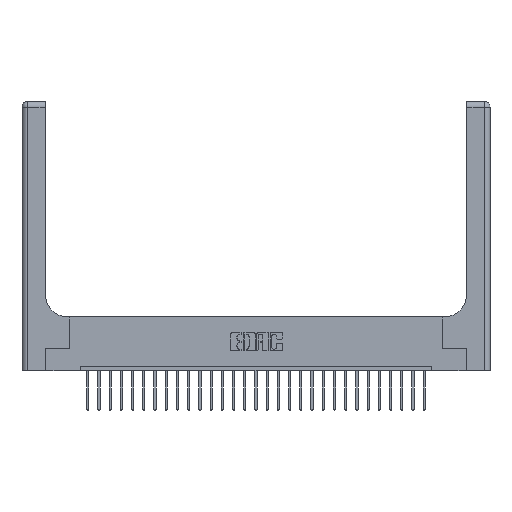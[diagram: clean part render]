
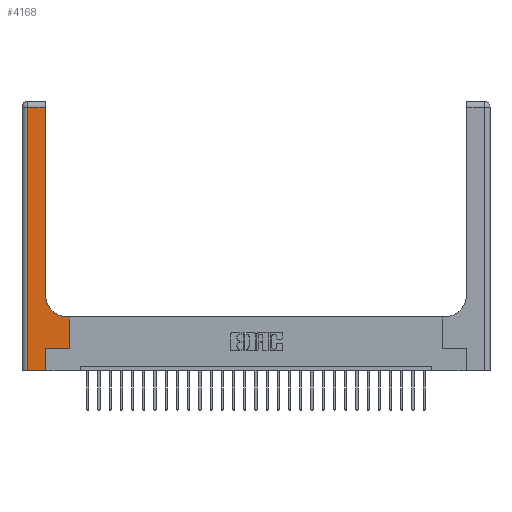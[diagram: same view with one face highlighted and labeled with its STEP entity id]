
A CAD part, top view. The second image highlights one B-rep face of the part: STEP entity #4168.
In plain terms, the highlighted planar face has unit normal (0, 0, 1).
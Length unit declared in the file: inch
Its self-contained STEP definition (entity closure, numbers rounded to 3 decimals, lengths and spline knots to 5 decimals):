
#510 = CARTESIAN_POINT ( 'NONE',  ( 0.26, 0.85, 0.37 ) ) ;
#938 = VERTEX_POINT ( 'NONE', #22805 ) ;
#1607 = LINE ( 'NONE', #25486, #23096 ) ;
#1623 = VECTOR ( 'NONE', #7981, 39.37008 ) ;
#1675 = DIRECTION ( 'NONE',  ( 0., 1., 0. ) ) ;
#1730 = CARTESIAN_POINT ( 'NONE',  ( 0., 0., 0.37 ) ) ;
#1995 = VERTEX_POINT ( 'NONE', #13888 ) ;
#2471 = DIRECTION ( 'NONE',  ( 0., 0., -1. ) ) ;
#3224 = VERTEX_POINT ( 'NONE', #7228 ) ;
#3388 = VERTEX_POINT ( 'NONE', #16816 ) ;
#3666 = CARTESIAN_POINT ( 'NONE',  ( 0.528, 0.25, 0.37 ) ) ;
#3952 = VERTEX_POINT ( 'NONE', #13189 ) ;
#4013 = CARTESIAN_POINT ( 'NONE',  ( 0.26, 0.6, 0.37 ) ) ;
#4091 = CARTESIAN_POINT ( 'NONE',  ( 0.26, 3., 0.37 ) ) ;
#4106 = EDGE_CURVE ( 'NONE', #938, #3388, #9564, .T. ) ;
#4168 = ADVANCED_FACE ( 'NONE', ( #8212 ), #18738, .F. ) ;
#5212 = DIRECTION ( 'NONE',  ( 1., 0., 0. ) ) ;
#5298 = EDGE_CURVE ( 'NONE', #1995, #7631, #5673, .T. ) ;
#5673 = LINE ( 'NONE', #19688, #8326 ) ;
#5877 = LINE ( 'NONE', #4013, #9491 ) ;
#6114 = VECTOR ( 'NONE', #1675, 39.37008 ) ;
#6427 = VERTEX_POINT ( 'NONE', #13700 ) ;
#6480 = EDGE_CURVE ( 'NONE', #9875, #25580, #8840, .T. ) ;
#7228 = CARTESIAN_POINT ( 'NONE',  ( 0.528, 0.25, 0.37 ) ) ;
#7511 = EDGE_CURVE ( 'NONE', #7631, #3952, #24387, .T. ) ;
#7631 = VERTEX_POINT ( 'NONE', #9044 ) ;
#7810 = DIRECTION ( 'NONE',  ( 0., 1., 0. ) ) ;
#7981 = DIRECTION ( 'NONE',  ( 0., -1., 0. ) ) ;
#8212 = FACE_OUTER_BOUND ( 'NONE', #10361, .T. ) ;
#8326 = VECTOR ( 'NONE', #15957, 39.37008 ) ;
#8474 = CARTESIAN_POINT ( 'NONE',  ( 0., 3., 0.37 ) ) ;
#8840 = CIRCLE ( 'NONE', #23749, 0.25 ) ;
#9044 = CARTESIAN_POINT ( 'NONE',  ( 0.06, 2.94, 0.37 ) ) ;
#9255 = EDGE_CURVE ( 'NONE', #25580, #1995, #10365, .T. ) ;
#9358 = VECTOR ( 'NONE', #22104, 39.37008 ) ;
#9491 = VECTOR ( 'NONE', #16160, 39.37008 ) ;
#9564 = LINE ( 'NONE', #26076, #21756 ) ;
#9875 = VERTEX_POINT ( 'NONE', #20998 ) ;
#10361 = EDGE_LOOP ( 'NONE', ( #24548, #23076, #20923, #11060, #18143, #10682, #15654, #11019, #11666 ) ) ;
#10365 = LINE ( 'NONE', #4091, #9358 ) ;
#10682 = ORIENTED_EDGE ( 'NONE', *, *, #14332, .T. ) ;
#11019 = ORIENTED_EDGE ( 'NONE', *, *, #20191, .T. ) ;
#11060 = ORIENTED_EDGE ( 'NONE', *, *, #25303, .T. ) ;
#11666 = ORIENTED_EDGE ( 'NONE', *, *, #6480, .T. ) ;
#11710 = DIRECTION ( 'NONE',  ( 1., 0., 0. ) ) ;
#11883 = DIRECTION ( 'NONE',  ( 1., 0., 0. ) ) ;
#11970 = CARTESIAN_POINT ( 'NONE',  ( 0.51, 0.85, 0.37 ) ) ;
#13189 = CARTESIAN_POINT ( 'NONE',  ( 0.06, 0., 0.37 ) ) ;
#13700 = CARTESIAN_POINT ( 'NONE',  ( 0.528, 0.6, 0.37 ) ) ;
#13888 = CARTESIAN_POINT ( 'NONE',  ( 0.26, 2.94, 0.37 ) ) ;
#14332 = EDGE_CURVE ( 'NONE', #3388, #3224, #1607, .T. ) ;
#15654 = ORIENTED_EDGE ( 'NONE', *, *, #20967, .T. ) ;
#15957 = DIRECTION ( 'NONE',  ( -1., 0., 0. ) ) ;
#16160 = DIRECTION ( 'NONE',  ( -1., 0., 0. ) ) ;
#16816 = CARTESIAN_POINT ( 'NONE',  ( 0.265, 0.25, 0.37 ) ) ;
#18143 = ORIENTED_EDGE ( 'NONE', *, *, #4106, .T. ) ;
#18482 = DIRECTION ( 'NONE',  ( -1., 0., 0. ) ) ;
#18738 = PLANE ( 'NONE',  #25971 ) ;
#19688 = CARTESIAN_POINT ( 'NONE',  ( 0., 2.94, 0.37 ) ) ;
#19948 = LINE ( 'NONE', #3666, #6114 ) ;
#20191 = EDGE_CURVE ( 'NONE', #6427, #9875, #5877, .T. ) ;
#20923 = ORIENTED_EDGE ( 'NONE', *, *, #7511, .T. ) ;
#20967 = EDGE_CURVE ( 'NONE', #3224, #6427, #19948, .T. ) ;
#20998 = CARTESIAN_POINT ( 'NONE',  ( 0.51, 0.6, 0.37 ) ) ;
#21756 = VECTOR ( 'NONE', #7810, 39.37008 ) ;
#22104 = DIRECTION ( 'NONE',  ( 0., 1., 0. ) ) ;
#22226 = DIRECTION ( 'NONE',  ( 0., 0., -1. ) ) ;
#22805 = CARTESIAN_POINT ( 'NONE',  ( 0.265, 0., 0.37 ) ) ;
#23076 = ORIENTED_EDGE ( 'NONE', *, *, #5298, .T. ) ;
#23096 = VECTOR ( 'NONE', #5212, 39.37008 ) ;
#23749 = AXIS2_PLACEMENT_3D ( 'NONE', #11970, #22226, #11710 ) ;
#24387 = LINE ( 'NONE', #26248, #1623 ) ;
#24548 = ORIENTED_EDGE ( 'NONE', *, *, #9255, .T. ) ;
#24941 = LINE ( 'NONE', #1730, #25772 ) ;
#25303 = EDGE_CURVE ( 'NONE', #3952, #938, #24941, .T. ) ;
#25486 = CARTESIAN_POINT ( 'NONE',  ( 0.265, 0.25, 0.37 ) ) ;
#25580 = VERTEX_POINT ( 'NONE', #510 ) ;
#25772 = VECTOR ( 'NONE', #11883, 39.37008 ) ;
#25971 = AXIS2_PLACEMENT_3D ( 'NONE', #8474, #2471, #18482 ) ;
#26076 = CARTESIAN_POINT ( 'NONE',  ( 0.265, 0., 0.37 ) ) ;
#26248 = CARTESIAN_POINT ( 'NONE',  ( 0.06, 3., 0.37 ) ) ;
